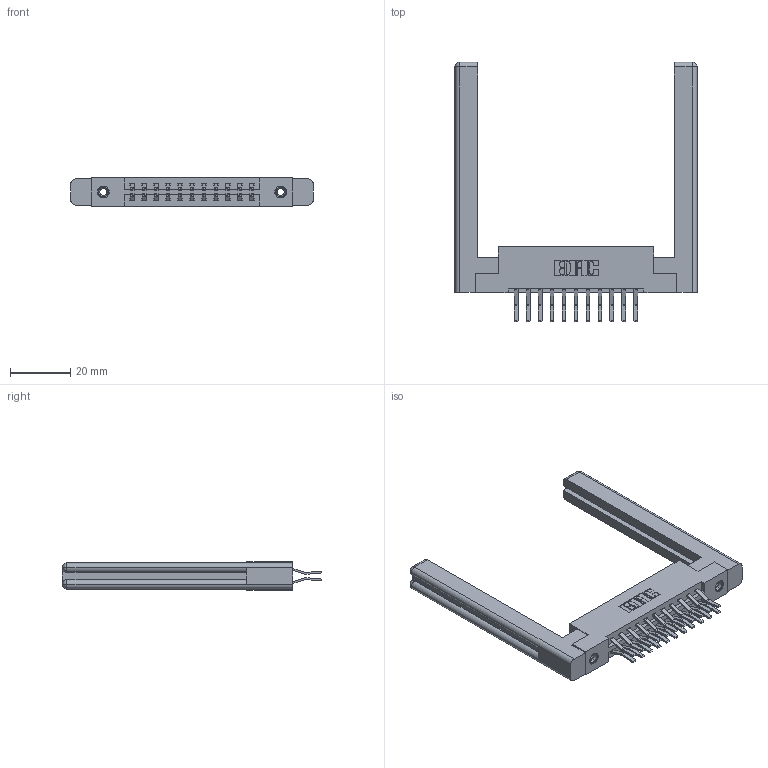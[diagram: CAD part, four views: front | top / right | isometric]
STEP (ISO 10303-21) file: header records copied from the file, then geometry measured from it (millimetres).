
FILE_DESCRIPTION (( 'STEP AP203' ), '1' );
FILE_NAME ('337-022-560-258.STEP', '2019-10-08T15:07:11', ( '' ), ( '' ), 'SwSTEP 2.0', 'SolidWorks 2016', '' );
FILE_SCHEMA (( 'CONFIG_CONTROL_DESIGN' ));
Length unit declared in the file: inch
Products named in the file (5): 307-220-058; 337 Part_Flush Mounting Lugs - 0.156 Dia-TI; 345-250-001_345-250-001-102; 337-022-560-258; 345-292-001_560 Tail
Assembly tree (27 placements, depth 2):
  337-022-560-258
    337 Part_Flush Mounting Lugs - 0.156 Dia-TI
    345-292-001_560 Tail  x22
    345-250-001_345-250-001-102  x2
    307-220-058  x2
Bounding box: 80.21 x 85.87 x 9.4 mm (x, y, z)
Volume: 15327.4 mm3; surface area: 14416.2 mm2
Topology: 27 solids, 27 shells, 1488 faces, 4339 edges, 2850 vertices
Faces by surface type: plane 990, cylinder 474, cone 12, torus 12
Entity records: 15260 total; most frequent: CARTESIAN_POINT 2605, ORIENTED_EDGE 2480, DIRECTION 2292, EDGE_CURVE 1240, VECTOR 1060, LINE 1060, VERTEX_POINT 818, AXIS2_PLACEMENT_3D 616
